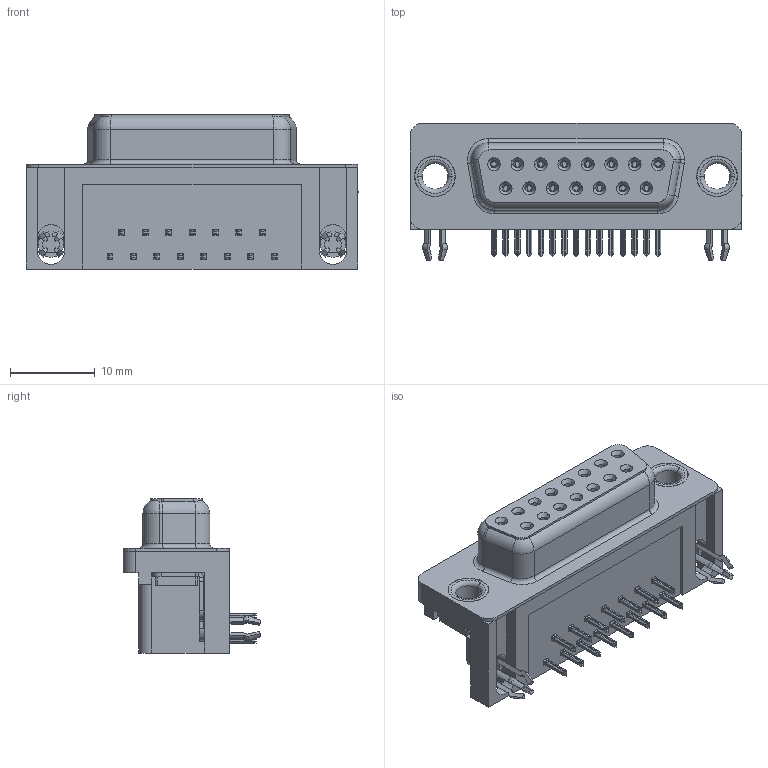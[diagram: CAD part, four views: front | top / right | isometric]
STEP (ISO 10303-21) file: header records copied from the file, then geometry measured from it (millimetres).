
FILE_DESCRIPTION (( 'STEP AP203' ), '1' );
FILE_NAME ('622-015-368-541.STEP', '2019-11-20T00:26:13', ( '' ), ( '' ), 'SwSTEP 2.0', 'SolidWorks 2016', '' );
FILE_SCHEMA (( 'CONFIG_CONTROL_DESIGN' ));
Length unit declared in the file: millimetre
Products named in the file (7): 622-015-368-541; 622 Housing_15 Socket; 622 Socket Bottom; 622 Shell_15 Socket; 622 Thru Hole Rivet; 622 4 Prong Board Lock; 622 Contact Top
Assembly tree (21 placements, depth 2):
  622-015-368-541
    622 Housing_15 Socket
    622 Shell_15 Socket
    622 Socket Bottom  x7
    622 Contact Top  x8
    622 4 Prong Board Lock  x2
    622 Thru Hole Rivet  x2
Bounding box: 39.22 x 16.25 x 18.2 mm (x, y, z)
Volume: 5185.2 mm3; surface area: 6766.9 mm2
Topology: 21 solids, 21 shells, 2507 faces, 6614 edges, 4164 vertices
Faces by surface type: plane 1116, cylinder 593, bspline 512, cone 220, torus 66
Entity records: 26265 total; most frequent: CARTESIAN_POINT 7488, ORIENTED_EDGE 3782, DIRECTION 3483, EDGE_CURVE 1891, VERTEX_POINT 1208, VECTOR 1163, LINE 1163, AXIS2_PLACEMENT_3D 1160
